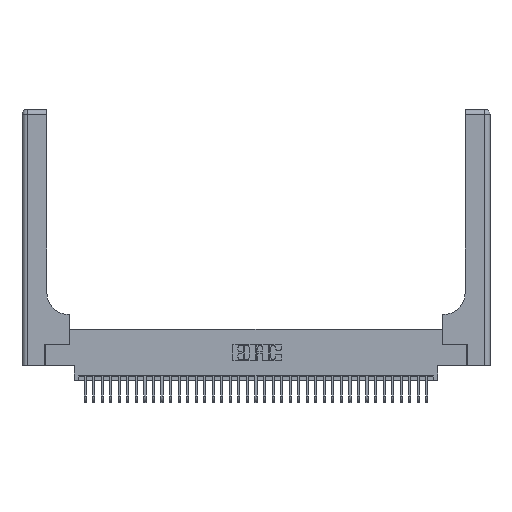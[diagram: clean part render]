
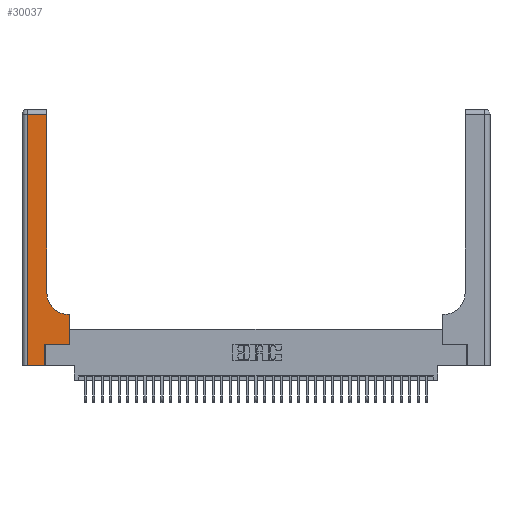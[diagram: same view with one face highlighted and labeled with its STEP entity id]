
A CAD part, top view. The second image highlights one B-rep face of the part: STEP entity #30037.
In plain terms, the highlighted planar face has unit normal (0, 0, 1).
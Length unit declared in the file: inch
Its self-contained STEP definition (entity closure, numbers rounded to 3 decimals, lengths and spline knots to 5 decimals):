
#369 = EDGE_CURVE ( 'NONE', #18374, #2433, #31124, .T. ) ;
#376 = CARTESIAN_POINT ( 'NONE',  ( 0.269, 0.25, 0.37 ) ) ;
#925 = EDGE_CURVE ( 'NONE', #35225, #10694, #4247, .T. ) ;
#936 = DIRECTION ( 'NONE',  ( -1., 0., 0. ) ) ;
#1378 = EDGE_CURVE ( 'NONE', #12427, #10508, #28449, .T. ) ;
#2433 = VERTEX_POINT ( 'NONE', #18101 ) ;
#2657 = VERTEX_POINT ( 'NONE', #10820 ) ;
#3202 = CARTESIAN_POINT ( 'NONE',  ( 0.2915, 3., 0.37 ) ) ;
#3235 = DIRECTION ( 'NONE',  ( -1., 0., 0. ) ) ;
#4247 = LINE ( 'NONE', #376, #33258 ) ;
#4311 = CARTESIAN_POINT ( 'NONE',  ( 0.5415, 0.6, 0.37 ) ) ;
#4427 = CARTESIAN_POINT ( 'NONE',  ( 0.269, 0., 0.37 ) ) ;
#4438 = CARTESIAN_POINT ( 'NONE',  ( 0.06, 0., 0.37 ) ) ;
#4719 = VECTOR ( 'NONE', #10615, 39.37008 ) ;
#4997 = VECTOR ( 'NONE', #24488, 39.37008 ) ;
#5385 = ORIENTED_EDGE ( 'NONE', *, *, #35377, .T. ) ;
#6073 = DIRECTION ( 'NONE',  ( 0., 1., 0. ) ) ;
#6113 = VECTOR ( 'NONE', #936, 39.37008 ) ;
#6547 = EDGE_CURVE ( 'NONE', #20642, #9199, #33201, .T. ) ;
#6710 = ORIENTED_EDGE ( 'NONE', *, *, #1378, .T. ) ;
#7473 = VECTOR ( 'NONE', #6073, 39.37008 ) ;
#7597 = VECTOR ( 'NONE', #13032, 39.37008 ) ;
#7641 = CARTESIAN_POINT ( 'NONE',  ( 0.269, 0., 0.37 ) ) ;
#8363 = CARTESIAN_POINT ( 'NONE',  ( 0.06, 2.94, 0.37 ) ) ;
#8468 = ORIENTED_EDGE ( 'NONE', *, *, #13050, .T. ) ;
#8915 = DIRECTION ( 'NONE',  ( 1., 0., 0. ) ) ;
#8945 = ORIENTED_EDGE ( 'NONE', *, *, #369, .T. ) ;
#9199 = VERTEX_POINT ( 'NONE', #8363 ) ;
#9539 = AXIS2_PLACEMENT_3D ( 'NONE', #14985, #34581, #17817 ) ;
#10508 = VERTEX_POINT ( 'NONE', #4427 ) ;
#10615 = DIRECTION ( 'NONE',  ( 0., 1., 0. ) ) ;
#10694 = VERTEX_POINT ( 'NONE', #30489 ) ;
#10820 = CARTESIAN_POINT ( 'NONE',  ( 0.5585, 0.6, 0.37 ) ) ;
#12427 = VERTEX_POINT ( 'NONE', #4438 ) ;
#12447 = ORIENTED_EDGE ( 'NONE', *, *, #13626, .T. ) ;
#12464 = CARTESIAN_POINT ( 'NONE',  ( 0.2915, 2.94, 0.37 ) ) ;
#12525 = LINE ( 'NONE', #7641, #4997 ) ;
#13032 = DIRECTION ( 'NONE',  ( 0., -1., 0. ) ) ;
#13050 = EDGE_CURVE ( 'NONE', #10508, #35225, #12525, .T. ) ;
#13626 = EDGE_CURVE ( 'NONE', #9199, #12427, #15096, .T. ) ;
#13708 = PLANE ( 'NONE',  #17871 ) ;
#14472 = LINE ( 'NONE', #23374, #6113 ) ;
#14985 = CARTESIAN_POINT ( 'NONE',  ( 0.5415, 0.85, 0.37 ) ) ;
#15096 = LINE ( 'NONE', #15723, #7597 ) ;
#15723 = CARTESIAN_POINT ( 'NONE',  ( 0.06, 3., 0.37 ) ) ;
#16091 = DIRECTION ( 'NONE',  ( 1., 0., 0. ) ) ;
#16540 = DIRECTION ( 'NONE',  ( 0., 0., -1. ) ) ;
#17817 = DIRECTION ( 'NONE',  ( 1., 0., 0. ) ) ;
#17871 = AXIS2_PLACEMENT_3D ( 'NONE', #30510, #16540, #36119 ) ;
#18101 = CARTESIAN_POINT ( 'NONE',  ( 0.2915, 0.85, 0.37 ) ) ;
#18357 = VECTOR ( 'NONE', #16091, 39.37008 ) ;
#18374 = VERTEX_POINT ( 'NONE', #4311 ) ;
#19212 = VECTOR ( 'NONE', #3235, 39.37008 ) ;
#20138 = CARTESIAN_POINT ( 'NONE',  ( 0., 2.94, 0.37 ) ) ;
#20373 = ORIENTED_EDGE ( 'NONE', *, *, #32580, .T. ) ;
#20642 = VERTEX_POINT ( 'NONE', #12464 ) ;
#21255 = CARTESIAN_POINT ( 'NONE',  ( 0.269, 0.25, 0.37 ) ) ;
#23374 = CARTESIAN_POINT ( 'NONE',  ( 0.2915, 0.6, 0.37 ) ) ;
#24488 = DIRECTION ( 'NONE',  ( 0., 1., 0. ) ) ;
#24724 = ORIENTED_EDGE ( 'NONE', *, *, #26704, .T. ) ;
#26704 = EDGE_CURVE ( 'NONE', #2433, #20642, #29898, .T. ) ;
#27008 = FACE_OUTER_BOUND ( 'NONE', #31633, .T. ) ;
#27168 = LINE ( 'NONE', #27439, #4719 ) ;
#27439 = CARTESIAN_POINT ( 'NONE',  ( 0.5585, 0.25, 0.37 ) ) ;
#28449 = LINE ( 'NONE', #35683, #18357 ) ;
#29898 = LINE ( 'NONE', #3202, #7473 ) ;
#30037 = ADVANCED_FACE ( 'NONE', ( #27008 ), #13708, .F. ) ;
#30489 = CARTESIAN_POINT ( 'NONE',  ( 0.5585, 0.25, 0.37 ) ) ;
#30510 = CARTESIAN_POINT ( 'NONE',  ( 0., 3., 0.37 ) ) ;
#31124 = CIRCLE ( 'NONE', #9539, 0.25 ) ;
#31633 = EDGE_LOOP ( 'NONE', ( #24724, #33919, #12447, #6710, #8468, #32616, #5385, #20373, #8945 ) ) ;
#32580 = EDGE_CURVE ( 'NONE', #2657, #18374, #14472, .T. ) ;
#32616 = ORIENTED_EDGE ( 'NONE', *, *, #925, .T. ) ;
#33201 = LINE ( 'NONE', #20138, #19212 ) ;
#33258 = VECTOR ( 'NONE', #8915, 39.37008 ) ;
#33919 = ORIENTED_EDGE ( 'NONE', *, *, #6547, .T. ) ;
#34581 = DIRECTION ( 'NONE',  ( 0., 0., -1. ) ) ;
#35225 = VERTEX_POINT ( 'NONE', #21255 ) ;
#35377 = EDGE_CURVE ( 'NONE', #10694, #2657, #27168, .T. ) ;
#35683 = CARTESIAN_POINT ( 'NONE',  ( 0., 0., 0.37 ) ) ;
#36119 = DIRECTION ( 'NONE',  ( -1., 0., 0. ) ) ;
